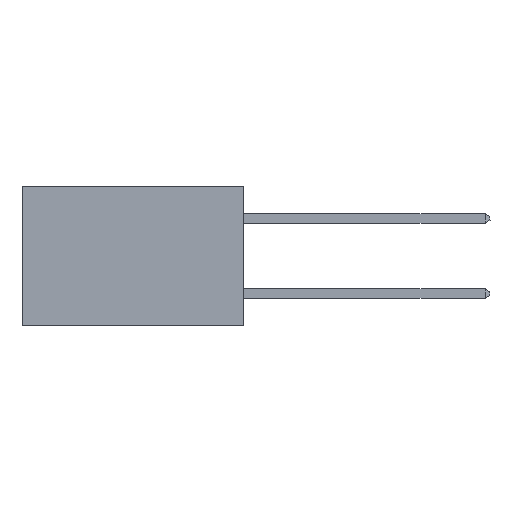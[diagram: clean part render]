
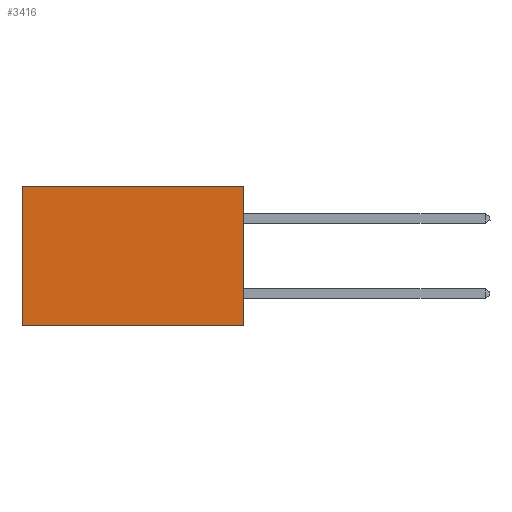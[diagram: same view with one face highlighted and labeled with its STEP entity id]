
A CAD part, left-side view. The second image highlights one B-rep face of the part: STEP entity #3416.
In plain terms, the highlighted planar face has unit normal (-1, 0, 0).
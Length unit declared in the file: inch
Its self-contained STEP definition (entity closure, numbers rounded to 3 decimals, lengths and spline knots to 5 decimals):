
#389 = VERTEX_POINT ( 'NONE', #8509 ) ;
#575 = VERTEX_POINT ( 'NONE', #7628 ) ;
#902 = CARTESIAN_POINT ( 'NONE',  ( 0.277, 0., -0.37 ) ) ;
#2347 = VERTEX_POINT ( 'NONE', #10396 ) ;
#2578 = EDGE_LOOP ( 'NONE', ( #6226, #8799, #3932, #6528 ) ) ;
#2740 = CARTESIAN_POINT ( 'NONE',  ( 0.277, 0.59, -0.37 ) ) ;
#2958 = VECTOR ( 'NONE', #7387, 39.37008 ) ;
#3212 = LINE ( 'NONE', #5243, #5300 ) ;
#3416 = ADVANCED_FACE ( 'NONE', ( #9160 ), #12112, .F. ) ;
#3932 = ORIENTED_EDGE ( 'NONE', *, *, #6695, .F. ) ;
#4355 = CARTESIAN_POINT ( 'NONE',  ( 0.277, 0., 0. ) ) ;
#4488 = EDGE_CURVE ( 'NONE', #2347, #575, #8785, .T. ) ;
#5243 = CARTESIAN_POINT ( 'NONE',  ( 0.277, 0., -0.37 ) ) ;
#5268 = DIRECTION ( 'NONE',  ( 0., 0., -1. ) ) ;
#5300 = VECTOR ( 'NONE', #5268, 39.37008 ) ;
#5862 = DIRECTION ( 'NONE',  ( 0., 1., 0. ) ) ;
#6049 = VERTEX_POINT ( 'NONE', #8069 ) ;
#6226 = ORIENTED_EDGE ( 'NONE', *, *, #4488, .T. ) ;
#6528 = ORIENTED_EDGE ( 'NONE', *, *, #8071, .T. ) ;
#6695 = EDGE_CURVE ( 'NONE', #389, #6049, #3212, .T. ) ;
#7335 = LINE ( 'NONE', #4355, #12104 ) ;
#7387 = DIRECTION ( 'NONE',  ( 0., 0., -1. ) ) ;
#7628 = CARTESIAN_POINT ( 'NONE',  ( 0.277, 0.59, -0.37 ) ) ;
#8069 = CARTESIAN_POINT ( 'NONE',  ( 0.277, 0., -0.37 ) ) ;
#8071 = EDGE_CURVE ( 'NONE', #389, #2347, #7335, .T. ) ;
#8137 = CARTESIAN_POINT ( 'NONE',  ( 0.277, 0., -0.37 ) ) ;
#8509 = CARTESIAN_POINT ( 'NONE',  ( 0.277, 0., 0. ) ) ;
#8583 = EDGE_CURVE ( 'NONE', #6049, #575, #12235, .T. ) ;
#8785 = LINE ( 'NONE', #2740, #2958 ) ;
#8799 = ORIENTED_EDGE ( 'NONE', *, *, #8583, .F. ) ;
#9116 = DIRECTION ( 'NONE',  ( 0., 1., 0. ) ) ;
#9160 = FACE_OUTER_BOUND ( 'NONE', #2578, .T. ) ;
#9581 = AXIS2_PLACEMENT_3D ( 'NONE', #8137, #12098, #12074 ) ;
#9946 = VECTOR ( 'NONE', #5862, 39.37008 ) ;
#10396 = CARTESIAN_POINT ( 'NONE',  ( 0.277, 0.59, 0. ) ) ;
#12074 = DIRECTION ( 'NONE',  ( 0., 0., -1. ) ) ;
#12098 = DIRECTION ( 'NONE',  ( 1., 0., 0. ) ) ;
#12104 = VECTOR ( 'NONE', #9116, 39.37008 ) ;
#12112 = PLANE ( 'NONE',  #9581 ) ;
#12235 = LINE ( 'NONE', #902, #9946 ) ;
